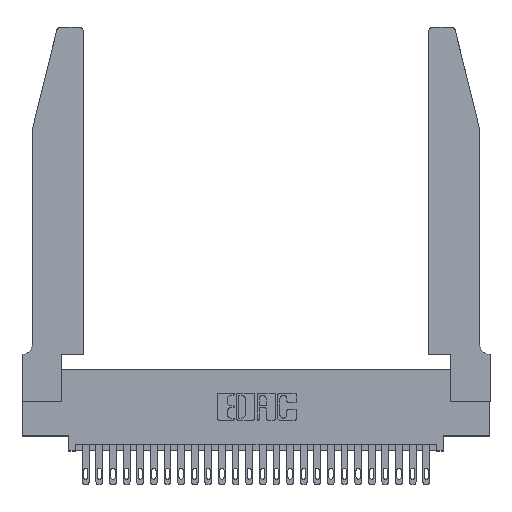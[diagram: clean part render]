
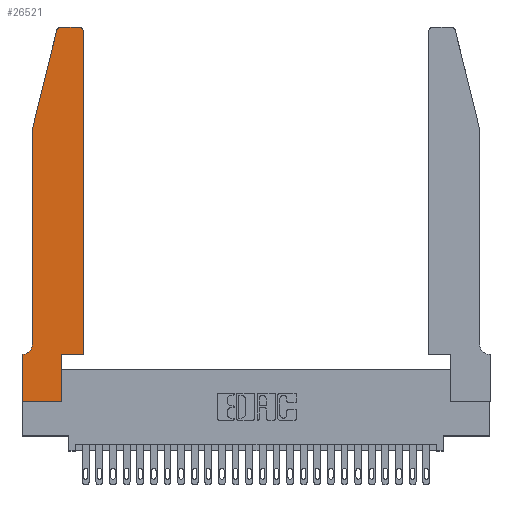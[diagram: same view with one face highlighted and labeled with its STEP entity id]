
A CAD part, top view. The second image highlights one B-rep face of the part: STEP entity #26521.
In plain terms, the highlighted planar face has unit normal (0, 0, 1).
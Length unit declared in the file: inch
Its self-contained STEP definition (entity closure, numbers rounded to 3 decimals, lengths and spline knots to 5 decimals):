
#48 = CARTESIAN_POINT ( 'NONE',  ( 0.4505, 0.35, 0.37 ) ) ;
#87 = LINE ( 'NONE', #7981, #4101 ) ;
#508 = CARTESIAN_POINT ( 'NONE',  ( 0.0755, 2., 0.37 ) ) ;
#530 = EDGE_CURVE ( 'NONE', #11295, #13410, #1176, .T. ) ;
#865 = VERTEX_POINT ( 'NONE', #12627 ) ;
#1061 = DIRECTION ( 'NONE',  ( -1., 0., 0. ) ) ;
#1176 = LINE ( 'NONE', #508, #16680 ) ;
#1424 = DIRECTION ( 'NONE',  ( 1., 0., 0. ) ) ;
#2143 = VERTEX_POINT ( 'NONE', #12114 ) ;
#2731 = LINE ( 'NONE', #17734, #27205 ) ;
#2873 = EDGE_LOOP ( 'NONE', ( #5262, #26189, #25358, #25566, #16951, #23552, #6387, #25241, #20488, #16800, #8459, #15717 ) ) ;
#2886 = CARTESIAN_POINT ( 'NONE',  ( 0.4505, 0.35, 0.37 ) ) ;
#3051 = CARTESIAN_POINT ( 'NONE',  ( 0.2605, 2.75, 0.37 ) ) ;
#4017 = CARTESIAN_POINT ( 'NONE',  ( 0.2865, 0., 0.37 ) ) ;
#4101 = VECTOR ( 'NONE', #10105, 39.37008 ) ;
#4715 = VERTEX_POINT ( 'NONE', #6337 ) ;
#4724 = VECTOR ( 'NONE', #14814, 39.37008 ) ;
#5002 = DIRECTION ( 'NONE',  ( 0., 0., -1. ) ) ;
#5218 = DIRECTION ( 'NONE',  ( -1., 0., 0. ) ) ;
#5262 = ORIENTED_EDGE ( 'NONE', *, *, #19997, .T. ) ;
#5627 = DIRECTION ( 'NONE',  ( 0., 0., 1. ) ) ;
#5656 = DIRECTION ( 'NONE',  ( 0., 0., 1. ) ) ;
#6337 = CARTESIAN_POINT ( 'NONE',  ( 0.4505, 2.72, 0.37 ) ) ;
#6378 = DIRECTION ( 'NONE',  ( 0., -1., 0. ) ) ;
#6387 = ORIENTED_EDGE ( 'NONE', *, *, #26621, .T. ) ;
#7247 = EDGE_CURVE ( 'NONE', #19328, #15276, #20193, .T. ) ;
#7685 = EDGE_CURVE ( 'NONE', #14026, #2143, #87, .T. ) ;
#7980 = DIRECTION ( 'NONE',  ( 1., 0., 0. ) ) ;
#7981 = CARTESIAN_POINT ( 'NONE',  ( 0.0755, 0.35, 0.37 ) ) ;
#8139 = EDGE_CURVE ( 'NONE', #25290, #11295, #2731, .T. ) ;
#8377 = AXIS2_PLACEMENT_3D ( 'NONE', #26213, #5002, #1061 ) ;
#8459 = ORIENTED_EDGE ( 'NONE', *, *, #22521, .T. ) ;
#8816 = AXIS2_PLACEMENT_3D ( 'NONE', #10006, #12228, #7980 ) ;
#8974 = CARTESIAN_POINT ( 'NONE',  ( 0.4205, 2.75, 0.37 ) ) ;
#9484 = CIRCLE ( 'NONE', #8816, 0.03 ) ;
#9642 = LINE ( 'NONE', #12546, #14565 ) ;
#9667 = CARTESIAN_POINT ( 'NONE',  ( 0.25487, 2.72718, 0.37 ) ) ;
#9680 = VECTOR ( 'NONE', #12658, 39.37008 ) ;
#9934 = VERTEX_POINT ( 'NONE', #23640 ) ;
#10003 = CARTESIAN_POINT ( 'NONE',  ( 0., 0., 0.37 ) ) ;
#10006 = CARTESIAN_POINT ( 'NONE',  ( 0.284, 2.72, 0.37 ) ) ;
#10028 = VERTEX_POINT ( 'NONE', #8974 ) ;
#10105 = DIRECTION ( 'NONE',  ( -1., 0., 0. ) ) ;
#11295 = VERTEX_POINT ( 'NONE', #13609 ) ;
#11855 = DIRECTION ( 'NONE',  ( 1., 0., 0. ) ) ;
#12114 = CARTESIAN_POINT ( 'NONE',  ( 0., 0.35, 0.37 ) ) ;
#12180 = PLANE ( 'NONE',  #26616 ) ;
#12228 = DIRECTION ( 'NONE',  ( 0., 0., 1. ) ) ;
#12546 = CARTESIAN_POINT ( 'NONE',  ( 0.2865, 0.35, 0.37 ) ) ;
#12627 = CARTESIAN_POINT ( 'NONE',  ( 0., 0., 0.37 ) ) ;
#12658 = DIRECTION ( 'NONE',  ( 1., 0., 0. ) ) ;
#12848 = EDGE_CURVE ( 'NONE', #4715, #10028, #21587, .T. ) ;
#13410 = VERTEX_POINT ( 'NONE', #22149 ) ;
#13609 = CARTESIAN_POINT ( 'NONE',  ( 0.0755, 2., 0.37 ) ) ;
#14026 = VERTEX_POINT ( 'NONE', #27045 ) ;
#14346 = DIRECTION ( 'NONE',  ( 1., 0., 0. ) ) ;
#14565 = VECTOR ( 'NONE', #18861, 39.37008 ) ;
#14814 = DIRECTION ( 'NONE',  ( 0., 1., 0. ) ) ;
#15067 = EDGE_CURVE ( 'NONE', #23584, #19328, #9642, .T. ) ;
#15276 = VERTEX_POINT ( 'NONE', #2886 ) ;
#15595 = DIRECTION ( 'NONE',  ( -0.239, -0.971, 0. ) ) ;
#15717 = ORIENTED_EDGE ( 'NONE', *, *, #12848, .T. ) ;
#16104 = VECTOR ( 'NONE', #11855, 39.37008 ) ;
#16498 = EDGE_CURVE ( 'NONE', #13410, #14026, #16628, .T. ) ;
#16628 = CIRCLE ( 'NONE', #8377, 0.07 ) ;
#16680 = VECTOR ( 'NONE', #26847, 39.37008 ) ;
#16800 = ORIENTED_EDGE ( 'NONE', *, *, #7247, .T. ) ;
#16951 = ORIENTED_EDGE ( 'NONE', *, *, #16498, .T. ) ;
#17273 = EDGE_CURVE ( 'NONE', #865, #23584, #23716, .T. ) ;
#17734 = CARTESIAN_POINT ( 'NONE',  ( 0.0755, 2., 0.37 ) ) ;
#17831 = AXIS2_PLACEMENT_3D ( 'NONE', #20573, #5627, #1424 ) ;
#18355 = FACE_OUTER_BOUND ( 'NONE', #2873, .T. ) ;
#18861 = DIRECTION ( 'NONE',  ( 0., 1., 0. ) ) ;
#19328 = VERTEX_POINT ( 'NONE', #19744 ) ;
#19657 = VECTOR ( 'NONE', #6378, 39.37008 ) ;
#19744 = CARTESIAN_POINT ( 'NONE',  ( 0.2865, 0.35, 0.37 ) ) ;
#19997 = EDGE_CURVE ( 'NONE', #10028, #9934, #21898, .T. ) ;
#20193 = LINE ( 'NONE', #23164, #9680 ) ;
#20246 = VECTOR ( 'NONE', #5218, 39.37008 ) ;
#20486 = LINE ( 'NONE', #48, #4724 ) ;
#20488 = ORIENTED_EDGE ( 'NONE', *, *, #15067, .T. ) ;
#20573 = CARTESIAN_POINT ( 'NONE',  ( 0.4205, 2.72, 0.37 ) ) ;
#21475 = EDGE_CURVE ( 'NONE', #9934, #25290, #9484, .T. ) ;
#21587 = CIRCLE ( 'NONE', #17831, 0.03 ) ;
#21898 = LINE ( 'NONE', #3051, #20246 ) ;
#22149 = CARTESIAN_POINT ( 'NONE',  ( 0.0755, 0.42, 0.37 ) ) ;
#22521 = EDGE_CURVE ( 'NONE', #15276, #4715, #20486, .T. ) ;
#23129 = CARTESIAN_POINT ( 'NONE',  ( 0., 0., 0.37 ) ) ;
#23164 = CARTESIAN_POINT ( 'NONE',  ( 0.4505, 0.35, 0.37 ) ) ;
#23552 = ORIENTED_EDGE ( 'NONE', *, *, #7685, .T. ) ;
#23584 = VERTEX_POINT ( 'NONE', #4017 ) ;
#23640 = CARTESIAN_POINT ( 'NONE',  ( 0.284, 2.75, 0.37 ) ) ;
#23716 = LINE ( 'NONE', #10003, #16104 ) ;
#25241 = ORIENTED_EDGE ( 'NONE', *, *, #17273, .T. ) ;
#25290 = VERTEX_POINT ( 'NONE', #9667 ) ;
#25358 = ORIENTED_EDGE ( 'NONE', *, *, #8139, .T. ) ;
#25566 = ORIENTED_EDGE ( 'NONE', *, *, #530, .T. ) ;
#26189 = ORIENTED_EDGE ( 'NONE', *, *, #21475, .T. ) ;
#26213 = CARTESIAN_POINT ( 'NONE',  ( 0.0055, 0.42, 0.37 ) ) ;
#26325 = LINE ( 'NONE', #23129, #19657 ) ;
#26521 = ADVANCED_FACE ( 'NONE', ( #18355 ), #12180, .T. ) ;
#26616 = AXIS2_PLACEMENT_3D ( 'NONE', #26946, #5656, #14346 ) ;
#26621 = EDGE_CURVE ( 'NONE', #2143, #865, #26325, .T. ) ;
#26847 = DIRECTION ( 'NONE',  ( 0., -1., 0. ) ) ;
#26946 = CARTESIAN_POINT ( 'NONE',  ( 0., 0.35, 0.37 ) ) ;
#27045 = CARTESIAN_POINT ( 'NONE',  ( 0.0055, 0.35, 0.37 ) ) ;
#27205 = VECTOR ( 'NONE', #15595, 39.37008 ) ;
